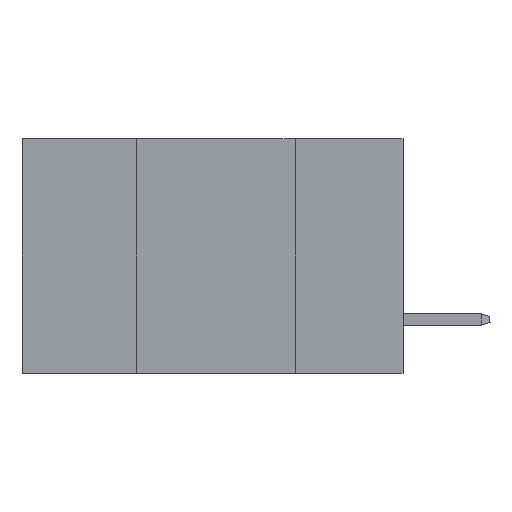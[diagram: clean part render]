
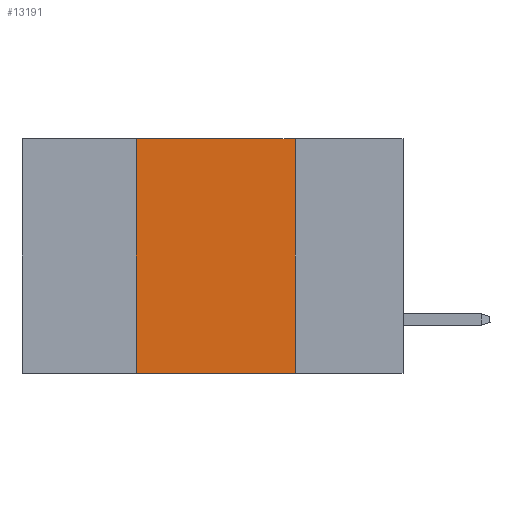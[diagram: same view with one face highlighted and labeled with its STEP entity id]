
A CAD part, left-side view. The second image highlights one B-rep face of the part: STEP entity #13191.
In plain terms, the highlighted planar face has unit normal (-1, 0, 0).
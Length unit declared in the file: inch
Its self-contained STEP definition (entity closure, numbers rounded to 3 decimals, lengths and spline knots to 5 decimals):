
#50 = LINE ( 'NONE', #15634, #11637 ) ;
#236 = VERTEX_POINT ( 'NONE', #20279 ) ;
#1334 = ORIENTED_EDGE ( 'NONE', *, *, #22340, .F. ) ;
#1520 = DIRECTION ( 'NONE',  ( 0., -1., 0. ) ) ;
#2484 = DIRECTION ( 'NONE',  ( 0., 0., -1. ) ) ;
#3761 = VECTOR ( 'NONE', #1520, 39.37008 ) ;
#3864 = CARTESIAN_POINT ( 'NONE',  ( 0., 0.6, -0.37 ) ) ;
#4449 = VECTOR ( 'NONE', #23726, 39.37008 ) ;
#6662 = EDGE_CURVE ( 'NONE', #19871, #236, #11780, .T. ) ;
#7780 = DIRECTION ( 'NONE',  ( 0., -1., 0. ) ) ;
#8644 = CARTESIAN_POINT ( 'NONE',  ( 0., 0.17, 0. ) ) ;
#9572 = DIRECTION ( 'NONE',  ( 0., 0., 1. ) ) ;
#10670 = VECTOR ( 'NONE', #7780, 39.37008 ) ;
#11637 = VECTOR ( 'NONE', #9572, 39.37008 ) ;
#11780 = LINE ( 'NONE', #21584, #4449 ) ;
#12238 = EDGE_CURVE ( 'NONE', #21288, #19871, #18875, .T. ) ;
#12482 = ORIENTED_EDGE ( 'NONE', *, *, #13349, .T. ) ;
#13191 = ADVANCED_FACE ( 'NONE', ( #22061 ), #18172, .F. ) ;
#13349 = EDGE_CURVE ( 'NONE', #18079, #236, #21149, .T. ) ;
#13532 = CARTESIAN_POINT ( 'NONE',  ( 0., 0.42, -0.37 ) ) ;
#14369 = CARTESIAN_POINT ( 'NONE',  ( 0., 0.6, 0. ) ) ;
#14824 = ORIENTED_EDGE ( 'NONE', *, *, #6662, .F. ) ;
#15634 = CARTESIAN_POINT ( 'NONE',  ( 0., 0.42, 0. ) ) ;
#17243 = CARTESIAN_POINT ( 'NONE',  ( 0., 0.6, 0. ) ) ;
#18079 = VERTEX_POINT ( 'NONE', #13532 ) ;
#18172 = PLANE ( 'NONE',  #23954 ) ;
#18531 = CARTESIAN_POINT ( 'NONE',  ( 0., 0.42, 0. ) ) ;
#18749 = ORIENTED_EDGE ( 'NONE', *, *, #12238, .F. ) ;
#18875 = LINE ( 'NONE', #17243, #3761 ) ;
#19017 = EDGE_LOOP ( 'NONE', ( #14824, #18749, #1334, #12482 ) ) ;
#19817 = DIRECTION ( 'NONE',  ( 1., 0., 0. ) ) ;
#19871 = VERTEX_POINT ( 'NONE', #8644 ) ;
#20279 = CARTESIAN_POINT ( 'NONE',  ( 0., 0.17, -0.37 ) ) ;
#21149 = LINE ( 'NONE', #3864, #10670 ) ;
#21288 = VERTEX_POINT ( 'NONE', #18531 ) ;
#21584 = CARTESIAN_POINT ( 'NONE',  ( 0., 0.17, 0. ) ) ;
#22061 = FACE_OUTER_BOUND ( 'NONE', #19017, .T. ) ;
#22340 = EDGE_CURVE ( 'NONE', #18079, #21288, #50, .T. ) ;
#23726 = DIRECTION ( 'NONE',  ( 0., 0., -1. ) ) ;
#23954 = AXIS2_PLACEMENT_3D ( 'NONE', #14369, #19817, #2484 ) ;
